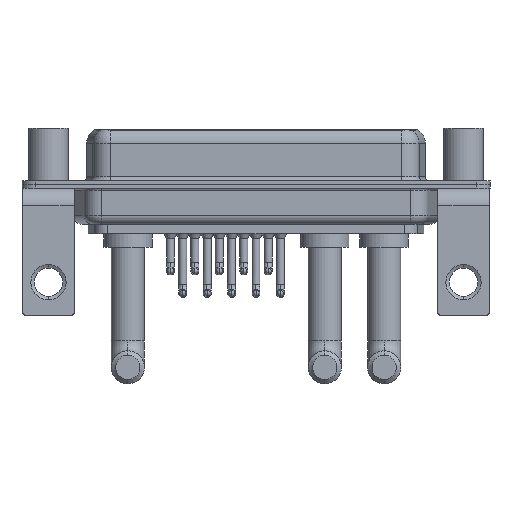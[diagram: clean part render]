
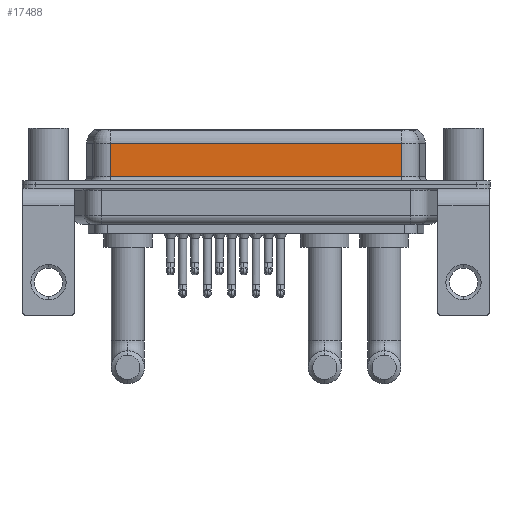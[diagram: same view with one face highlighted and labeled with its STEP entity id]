
A CAD part, front view. The second image highlights one B-rep face of the part: STEP entity #17488.
In plain terms, the highlighted planar face has unit normal (0, -1, 0).
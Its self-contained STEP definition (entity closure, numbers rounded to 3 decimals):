
#1066 = DIRECTION ( 'NONE',  ( 0., 0., -1. ) ) ;
#1809 = CARTESIAN_POINT ( 'NONE',  ( 40.037, -3.95, 6.4 ) ) ;
#1856 = CARTESIAN_POINT ( 'NONE',  ( 40.037, -3.95, 0.9 ) ) ;
#1944 = CARTESIAN_POINT ( 'NONE',  ( 7.013, -3.95, 6.4 ) ) ;
#2197 = EDGE_LOOP ( 'NONE', ( #9121, #7227, #4729, #6451 ) ) ;
#3195 = CARTESIAN_POINT ( 'NONE',  ( 40.037, -3.95, 4.65 ) ) ;
#4641 = DIRECTION ( 'NONE',  ( 0., 0., 1. ) ) ;
#4729 = ORIENTED_EDGE ( 'NONE', *, *, #17019, .T. ) ;
#6451 = ORIENTED_EDGE ( 'NONE', *, *, #20149, .T. ) ;
#7227 = ORIENTED_EDGE ( 'NONE', *, *, #14709, .T. ) ;
#8000 = CARTESIAN_POINT ( 'NONE',  ( 40.037, -3.95, 4.65 ) ) ;
#8066 = VECTOR ( 'NONE', #9915, 1000. ) ;
#8287 = VECTOR ( 'NONE', #20389, 1000. ) ;
#8318 = DIRECTION ( 'NONE',  ( -1., 0., 0. ) ) ;
#9121 = ORIENTED_EDGE ( 'NONE', *, *, #20968, .F. ) ;
#9151 = CARTESIAN_POINT ( 'NONE',  ( 40.037, -3.95, 0.9 ) ) ;
#9915 = DIRECTION ( 'NONE',  ( 1., 0., 0. ) ) ;
#11084 = LINE ( 'NONE', #14162, #17117 ) ;
#11616 = FACE_OUTER_BOUND ( 'NONE', #2197, .T. ) ;
#12874 = VERTEX_POINT ( 'NONE', #3195 ) ;
#14162 = CARTESIAN_POINT ( 'NONE',  ( 40.037, -3.95, 6.4 ) ) ;
#14598 = DIRECTION ( 'NONE',  ( 0., 1., 0. ) ) ;
#14709 = EDGE_CURVE ( 'NONE', #12874, #21244, #14998, .T. ) ;
#14936 = VERTEX_POINT ( 'NONE', #9151 ) ;
#14998 = LINE ( 'NONE', #8000, #19796 ) ;
#16030 = VERTEX_POINT ( 'NONE', #19012 ) ;
#16327 = AXIS2_PLACEMENT_3D ( 'NONE', #1809, #14598, #4641 ) ;
#16755 = PLANE ( 'NONE',  #16327 ) ;
#16888 = LINE ( 'NONE', #1944, #8287 ) ;
#17019 = EDGE_CURVE ( 'NONE', #21244, #16030, #16888, .T. ) ;
#17117 = VECTOR ( 'NONE', #1066, 1000. ) ;
#17293 = CARTESIAN_POINT ( 'NONE',  ( 7.013, -3.95, 4.65 ) ) ;
#17488 = ADVANCED_FACE ( 'NONE', ( #11616 ), #16755, .F. ) ;
#18441 = LINE ( 'NONE', #1856, #8066 ) ;
#19012 = CARTESIAN_POINT ( 'NONE',  ( 7.013, -3.95, 0.9 ) ) ;
#19796 = VECTOR ( 'NONE', #8318, 1000. ) ;
#20149 = EDGE_CURVE ( 'NONE', #16030, #14936, #18441, .T. ) ;
#20389 = DIRECTION ( 'NONE',  ( 0., 0., -1. ) ) ;
#20968 = EDGE_CURVE ( 'NONE', #12874, #14936, #11084, .T. ) ;
#21244 = VERTEX_POINT ( 'NONE', #17293 ) ;
